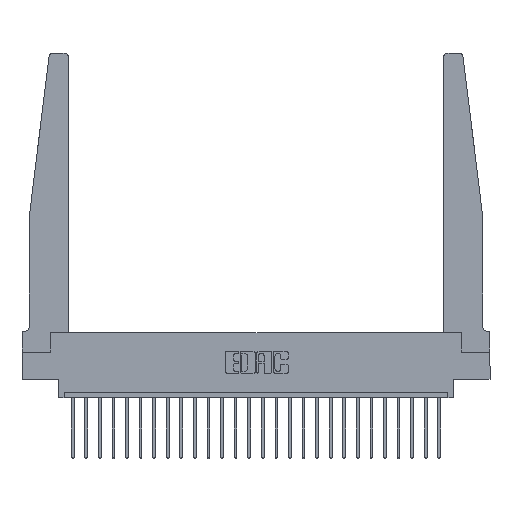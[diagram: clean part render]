
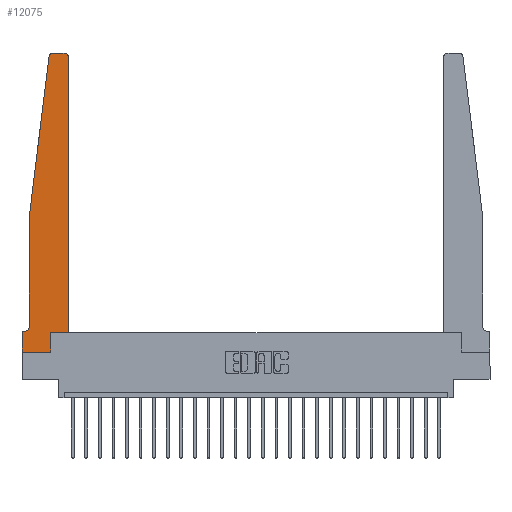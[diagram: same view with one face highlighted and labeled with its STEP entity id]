
A CAD part, top view. The second image highlights one B-rep face of the part: STEP entity #12075.
In plain terms, the highlighted planar face has unit normal (0, 0, 1).
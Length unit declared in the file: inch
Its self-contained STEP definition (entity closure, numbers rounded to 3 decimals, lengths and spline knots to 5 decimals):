
#210 = VECTOR ( 'NONE', #21983, 39.37008 ) ;
#214 = DIRECTION ( 'NONE',  ( 0., 1., 0. ) ) ;
#592 = VERTEX_POINT ( 'NONE', #15602 ) ;
#1134 = EDGE_CURVE ( 'NONE', #7597, #17100, #10278, .T. ) ;
#1233 = CIRCLE ( 'NONE', #19168, 0.03 ) ;
#1320 = EDGE_CURVE ( 'NONE', #21116, #14071, #9403, .T. ) ;
#1330 = CARTESIAN_POINT ( 'NONE',  ( 0.425, 0.18, 0.37 ) ) ;
#1537 = CARTESIAN_POINT ( 'NONE',  ( 0.27653, 2.72, 0.37 ) ) ;
#1802 = DIRECTION ( 'NONE',  ( 1., 0., 0. ) ) ;
#2099 = VECTOR ( 'NONE', #1802, 39.37008 ) ;
#2469 = VERTEX_POINT ( 'NONE', #17170 ) ;
#2509 = ORIENTED_EDGE ( 'NONE', *, *, #7467, .T. ) ;
#2636 = VECTOR ( 'NONE', #17411, 39.37008 ) ;
#2645 = VERTEX_POINT ( 'NONE', #5211 ) ;
#3208 = DIRECTION ( 'NONE',  ( 0., 1., 0. ) ) ;
#3288 = LINE ( 'NONE', #20689, #16461 ) ;
#3717 = EDGE_CURVE ( 'NONE', #592, #14648, #20617, .T. ) ;
#3913 = ORIENTED_EDGE ( 'NONE', *, *, #3717, .T. ) ;
#4022 = DIRECTION ( 'NONE',  ( 1., 0., 0. ) ) ;
#4540 = EDGE_CURVE ( 'NONE', #8014, #592, #7182, .T. ) ;
#4562 = VERTEX_POINT ( 'NONE', #22703 ) ;
#5061 = DIRECTION ( 'NONE',  ( 0., 0., 1. ) ) ;
#5089 = ORIENTED_EDGE ( 'NONE', *, *, #18697, .T. ) ;
#5174 = CARTESIAN_POINT ( 'NONE',  ( 0.065, 1.25, 0.37 ) ) ;
#5211 = CARTESIAN_POINT ( 'NONE',  ( 0.2605, 0., 0.37 ) ) ;
#5245 = DIRECTION ( 'NONE',  ( -1., 0., 0. ) ) ;
#5636 = CARTESIAN_POINT ( 'NONE',  ( 0.395, 2.72, 0.37 ) ) ;
#5786 = VECTOR ( 'NONE', #16351, 39.37008 ) ;
#5897 = EDGE_CURVE ( 'NONE', #2645, #21116, #18254, .T. ) ;
#6411 = ORIENTED_EDGE ( 'NONE', *, *, #12281, .T. ) ;
#6464 = ORIENTED_EDGE ( 'NONE', *, *, #4540, .T. ) ;
#6977 = CARTESIAN_POINT ( 'NONE',  ( 0.015, 0.1875, 0.37 ) ) ;
#7182 = LINE ( 'NONE', #5174, #8639 ) ;
#7462 = VECTOR ( 'NONE', #214, 39.37008 ) ;
#7467 = EDGE_CURVE ( 'NONE', #4562, #8014, #3288, .T. ) ;
#7597 = VERTEX_POINT ( 'NONE', #19055 ) ;
#8014 = VERTEX_POINT ( 'NONE', #16462 ) ;
#8433 = CIRCLE ( 'NONE', #13179, 0.03 ) ;
#8639 = VECTOR ( 'NONE', #16656, 39.37008 ) ;
#8961 = EDGE_CURVE ( 'NONE', #14071, #2469, #12912, .T. ) ;
#9087 = CARTESIAN_POINT ( 'NONE',  ( 0., 0., 0.37 ) ) ;
#9205 = PLANE ( 'NONE',  #11920 ) ;
#9328 = CARTESIAN_POINT ( 'NONE',  ( 0.25, 2.75, 0.37 ) ) ;
#9403 = LINE ( 'NONE', #16185, #2636 ) ;
#9576 = DIRECTION ( 'NONE',  ( -0.122, -0.992, 0. ) ) ;
#9608 = LINE ( 'NONE', #10771, #5786 ) ;
#9906 = LINE ( 'NONE', #20091, #210 ) ;
#10278 = LINE ( 'NONE', #9328, #18728 ) ;
#10403 = CARTESIAN_POINT ( 'NONE',  ( 0., 0., 0.37 ) ) ;
#10758 = CARTESIAN_POINT ( 'NONE',  ( 0.425, 0.18, 0.37 ) ) ;
#10771 = CARTESIAN_POINT ( 'NONE',  ( 0., 0., 0.37 ) ) ;
#11078 = DIRECTION ( 'NONE',  ( 0., 0., 1. ) ) ;
#11545 = CARTESIAN_POINT ( 'NONE',  ( 0.27653, 2.75, 0.37 ) ) ;
#11795 = VERTEX_POINT ( 'NONE', #12839 ) ;
#11838 = EDGE_CURVE ( 'NONE', #2469, #7597, #8433, .T. ) ;
#11920 = AXIS2_PLACEMENT_3D ( 'NONE', #22211, #11078, #4022 ) ;
#12075 = ADVANCED_FACE ( 'NONE', ( #23871 ), #9205, .T. ) ;
#12281 = EDGE_CURVE ( 'NONE', #14648, #11795, #9906, .T. ) ;
#12382 = ORIENTED_EDGE ( 'NONE', *, *, #18950, .T. ) ;
#12839 = CARTESIAN_POINT ( 'NONE',  ( 0., 0.1875, 0.37 ) ) ;
#12912 = LINE ( 'NONE', #1330, #15540 ) ;
#13179 = AXIS2_PLACEMENT_3D ( 'NONE', #5636, #22588, #15058 ) ;
#13461 = DIRECTION ( 'NONE',  ( -1., 0., 0. ) ) ;
#14071 = VERTEX_POINT ( 'NONE', #10758 ) ;
#14477 = CARTESIAN_POINT ( 'NONE',  ( 0.015, 0.2375, 0.37 ) ) ;
#14529 = DIRECTION ( 'NONE',  ( 1., 0., 0. ) ) ;
#14642 = ORIENTED_EDGE ( 'NONE', *, *, #11838, .T. ) ;
#14648 = VERTEX_POINT ( 'NONE', #6977 ) ;
#15058 = DIRECTION ( 'NONE',  ( 1., 0., 0. ) ) ;
#15205 = CARTESIAN_POINT ( 'NONE',  ( 0.2605, 0.18, 0.37 ) ) ;
#15540 = VECTOR ( 'NONE', #3208, 39.37008 ) ;
#15602 = CARTESIAN_POINT ( 'NONE',  ( 0.065, 0.2375, 0.37 ) ) ;
#16185 = CARTESIAN_POINT ( 'NONE',  ( 0.425, 0.18, 0.37 ) ) ;
#16351 = DIRECTION ( 'NONE',  ( 0., -1., 0. ) ) ;
#16455 = DIRECTION ( 'NONE',  ( 0., 0., -1. ) ) ;
#16461 = VECTOR ( 'NONE', #9576, 39.37008 ) ;
#16462 = CARTESIAN_POINT ( 'NONE',  ( 0.065, 1.25, 0.37 ) ) ;
#16656 = DIRECTION ( 'NONE',  ( 0., -1., 0. ) ) ;
#16763 = LINE ( 'NONE', #9087, #2099 ) ;
#17100 = VERTEX_POINT ( 'NONE', #11545 ) ;
#17170 = CARTESIAN_POINT ( 'NONE',  ( 0.425, 2.72, 0.37 ) ) ;
#17245 = EDGE_LOOP ( 'NONE', ( #21521, #12382, #2509, #6464, #3913, #6411, #23367, #5089, #19612, #21633, #23725, #14642 ) ) ;
#17411 = DIRECTION ( 'NONE',  ( 1., 0., 0. ) ) ;
#18254 = LINE ( 'NONE', #15205, #7462 ) ;
#18697 = EDGE_CURVE ( 'NONE', #21834, #2645, #16763, .T. ) ;
#18728 = VECTOR ( 'NONE', #13461, 39.37008 ) ;
#18950 = EDGE_CURVE ( 'NONE', #17100, #4562, #1233, .T. ) ;
#19055 = CARTESIAN_POINT ( 'NONE',  ( 0.395, 2.75, 0.37 ) ) ;
#19168 = AXIS2_PLACEMENT_3D ( 'NONE', #1537, #5061, #14529 ) ;
#19612 = ORIENTED_EDGE ( 'NONE', *, *, #5897, .T. ) ;
#20091 = CARTESIAN_POINT ( 'NONE',  ( 0.065, 0.1875, 0.37 ) ) ;
#20617 = CIRCLE ( 'NONE', #21770, 0.05 ) ;
#20689 = CARTESIAN_POINT ( 'NONE',  ( 0.065, 1.25, 0.37 ) ) ;
#21045 = EDGE_CURVE ( 'NONE', #11795, #21834, #9608, .T. ) ;
#21116 = VERTEX_POINT ( 'NONE', #23493 ) ;
#21521 = ORIENTED_EDGE ( 'NONE', *, *, #1134, .T. ) ;
#21633 = ORIENTED_EDGE ( 'NONE', *, *, #1320, .T. ) ;
#21770 = AXIS2_PLACEMENT_3D ( 'NONE', #14477, #16455, #5245 ) ;
#21834 = VERTEX_POINT ( 'NONE', #10403 ) ;
#21983 = DIRECTION ( 'NONE',  ( -1., 0., 0. ) ) ;
#22211 = CARTESIAN_POINT ( 'NONE',  ( 0., 0.1875, 0.37 ) ) ;
#22588 = DIRECTION ( 'NONE',  ( 0., 0., 1. ) ) ;
#22703 = CARTESIAN_POINT ( 'NONE',  ( 0.24675, 2.72367, 0.37 ) ) ;
#23367 = ORIENTED_EDGE ( 'NONE', *, *, #21045, .T. ) ;
#23493 = CARTESIAN_POINT ( 'NONE',  ( 0.2605, 0.18, 0.37 ) ) ;
#23725 = ORIENTED_EDGE ( 'NONE', *, *, #8961, .T. ) ;
#23871 = FACE_OUTER_BOUND ( 'NONE', #17245, .T. ) ;
